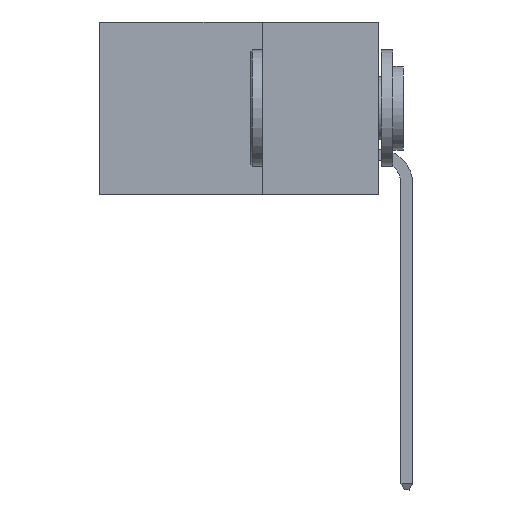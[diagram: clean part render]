
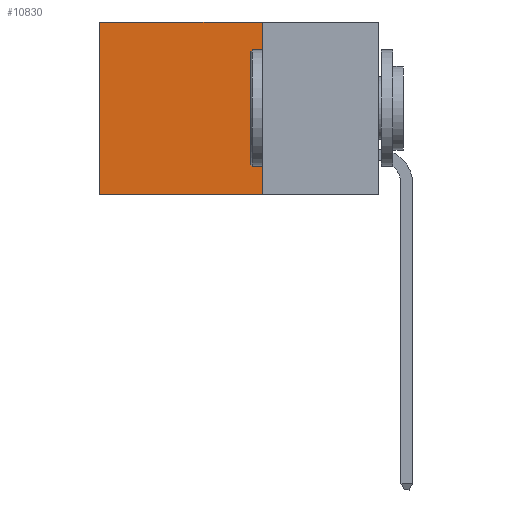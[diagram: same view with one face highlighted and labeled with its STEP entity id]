
A CAD part, left-side view. The second image highlights one B-rep face of the part: STEP entity #10830.
In plain terms, the highlighted planar face has unit normal (-1, 0, 0).
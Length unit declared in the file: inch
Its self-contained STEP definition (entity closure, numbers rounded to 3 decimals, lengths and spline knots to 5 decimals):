
#1562 = CARTESIAN_POINT ( 'NONE',  ( 0.298, 0.25, 0. ) ) ;
#3138 = VERTEX_POINT ( 'NONE', #26737 ) ;
#4909 = ORIENTED_EDGE ( 'NONE', *, *, #20392, .F. ) ;
#4916 = DIRECTION ( 'NONE',  ( 0., 1., 0. ) ) ;
#5012 = VECTOR ( 'NONE', #13122, 39.37008 ) ;
#5409 = DIRECTION ( 'NONE',  ( 0., 0., -1. ) ) ;
#6382 = LINE ( 'NONE', #26302, #22389 ) ;
#6563 = DIRECTION ( 'NONE',  ( 1., 0., 0. ) ) ;
#8556 = VERTEX_POINT ( 'NONE', #24174 ) ;
#8761 = VECTOR ( 'NONE', #12427, 39.37008 ) ;
#9845 = EDGE_LOOP ( 'NONE', ( #16737, #23387, #4909, #14034 ) ) ;
#9853 = AXIS2_PLACEMENT_3D ( 'NONE', #12567, #6563, #20870 ) ;
#10519 = LINE ( 'NONE', #15026, #5012 ) ;
#10830 = ADVANCED_FACE ( 'NONE', ( #25198 ), #14361, .F. ) ;
#10862 = CARTESIAN_POINT ( 'NONE',  ( 0.298, 0.6, -0.37 ) ) ;
#10919 = CARTESIAN_POINT ( 'NONE',  ( 0.298, 0.25, -0.37 ) ) ;
#12427 = DIRECTION ( 'NONE',  ( 0., 0., -1. ) ) ;
#12567 = CARTESIAN_POINT ( 'NONE',  ( 0.298, 0.25, 0. ) ) ;
#13122 = DIRECTION ( 'NONE',  ( 0., 1., 0. ) ) ;
#14034 = ORIENTED_EDGE ( 'NONE', *, *, #21780, .T. ) ;
#14150 = LINE ( 'NONE', #10919, #18721 ) ;
#14361 = PLANE ( 'NONE',  #9853 ) ;
#15026 = CARTESIAN_POINT ( 'NONE',  ( 0.298, 0.25, 0. ) ) ;
#15840 = EDGE_CURVE ( 'NONE', #3138, #20781, #18548, .T. ) ;
#16737 = ORIENTED_EDGE ( 'NONE', *, *, #15840, .T. ) ;
#18478 = CARTESIAN_POINT ( 'NONE',  ( 0.298, 0.6, 0. ) ) ;
#18548 = LINE ( 'NONE', #18478, #8761 ) ;
#18598 = EDGE_CURVE ( 'NONE', #8556, #20781, #14150, .T. ) ;
#18721 = VECTOR ( 'NONE', #4916, 39.37008 ) ;
#19078 = VERTEX_POINT ( 'NONE', #1562 ) ;
#20392 = EDGE_CURVE ( 'NONE', #19078, #8556, #6382, .T. ) ;
#20781 = VERTEX_POINT ( 'NONE', #10862 ) ;
#20870 = DIRECTION ( 'NONE',  ( 0., 0., -1. ) ) ;
#21780 = EDGE_CURVE ( 'NONE', #19078, #3138, #10519, .T. ) ;
#22389 = VECTOR ( 'NONE', #5409, 39.37008 ) ;
#23387 = ORIENTED_EDGE ( 'NONE', *, *, #18598, .F. ) ;
#24174 = CARTESIAN_POINT ( 'NONE',  ( 0.298, 0.25, -0.37 ) ) ;
#25198 = FACE_OUTER_BOUND ( 'NONE', #9845, .T. ) ;
#26302 = CARTESIAN_POINT ( 'NONE',  ( 0.298, 0.25, 0. ) ) ;
#26737 = CARTESIAN_POINT ( 'NONE',  ( 0.298, 0.6, 0. ) ) ;
